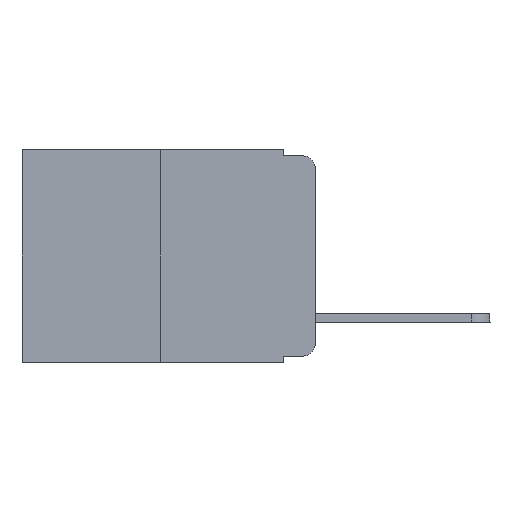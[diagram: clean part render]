
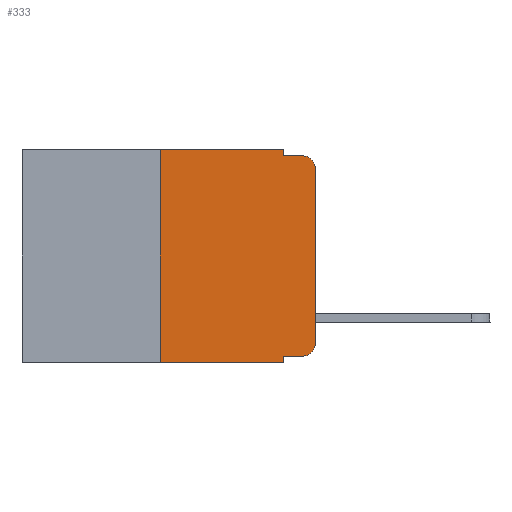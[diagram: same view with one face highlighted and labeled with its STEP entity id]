
A CAD part, left-side view. The second image highlights one B-rep face of the part: STEP entity #333.
In plain terms, the highlighted planar face has unit normal (-1, 0, 0).
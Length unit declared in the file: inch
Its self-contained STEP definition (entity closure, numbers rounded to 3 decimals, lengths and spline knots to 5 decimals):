
#112 = LINE ( 'NONE', #10300, #6305 ) ;
#148 = CARTESIAN_POINT ( 'NONE',  ( 0., 0.473, 0. ) ) ;
#184 = CARTESIAN_POINT ( 'NONE',  ( 0., 0.02, -0.313 ) ) ;
#333 = ADVANCED_FACE ( 'NONE', ( #2467 ), #12265, .F. ) ;
#410 = VECTOR ( 'NONE', #12248, 39.37008 ) ;
#501 = EDGE_CURVE ( 'NONE', #10799, #5024, #112, .T. ) ;
#825 = VECTOR ( 'NONE', #7896, 39.37008 ) ;
#920 = EDGE_CURVE ( 'NONE', #13143, #12940, #6471, .T. ) ;
#958 = CARTESIAN_POINT ( 'NONE',  ( 0., 0.02, -0.333 ) ) ;
#990 = DIRECTION ( 'NONE',  ( 0., 0., -1. ) ) ;
#1662 = LINE ( 'NONE', #13564, #9919 ) ;
#1767 = VERTEX_POINT ( 'NONE', #10139 ) ;
#1808 = CIRCLE ( 'NONE', #14668, 0.02 ) ;
#1961 = CARTESIAN_POINT ( 'NONE',  ( 0., 0.051, -0.01 ) ) ;
#2074 = ORIENTED_EDGE ( 'NONE', *, *, #2558, .T. ) ;
#2287 = VERTEX_POINT ( 'NONE', #15857 ) ;
#2348 = EDGE_CURVE ( 'NONE', #12079, #1767, #2848, .T. ) ;
#2377 = CIRCLE ( 'NONE', #14820, 0.02 ) ;
#2427 = LINE ( 'NONE', #7801, #11066 ) ;
#2467 = FACE_OUTER_BOUND ( 'NONE', #6230, .T. ) ;
#2558 = EDGE_CURVE ( 'NONE', #12079, #7260, #1662, .T. ) ;
#2848 = LINE ( 'NONE', #14008, #4174 ) ;
#3123 = DIRECTION ( 'NONE',  ( 0., 0., -1. ) ) ;
#3157 = LINE ( 'NONE', #14130, #825 ) ;
#3740 = LINE ( 'NONE', #7368, #410 ) ;
#3996 = DIRECTION ( 'NONE',  ( 0., 0., -1. ) ) ;
#4174 = VECTOR ( 'NONE', #10405, 39.37008 ) ;
#4663 = EDGE_CURVE ( 'NONE', #2287, #5148, #3157, .T. ) ;
#4719 = CARTESIAN_POINT ( 'NONE',  ( 0., 0.02, -0.03 ) ) ;
#4754 = VECTOR ( 'NONE', #7953, 39.37008 ) ;
#4758 = EDGE_CURVE ( 'NONE', #12940, #11638, #2377, .T. ) ;
#4834 = CARTESIAN_POINT ( 'NONE',  ( 0., 0., -0.03 ) ) ;
#4956 = AXIS2_PLACEMENT_3D ( 'NONE', #148, #6360, #8750 ) ;
#5024 = VERTEX_POINT ( 'NONE', #1961 ) ;
#5148 = VERTEX_POINT ( 'NONE', #958 ) ;
#5492 = CARTESIAN_POINT ( 'NONE',  ( 0., 0., -0.313 ) ) ;
#6230 = EDGE_LOOP ( 'NONE', ( #7452, #14135, #14355, #7091, #9943, #14234, #2074, #13016, #6827, #6243 ) ) ;
#6243 = ORIENTED_EDGE ( 'NONE', *, *, #8329, .T. ) ;
#6305 = VECTOR ( 'NONE', #3123, 39.37008 ) ;
#6360 = DIRECTION ( 'NONE',  ( 1., 0., 0. ) ) ;
#6457 = DIRECTION ( 'NONE',  ( -1., 0., 0. ) ) ;
#6471 = LINE ( 'NONE', #14773, #12975 ) ;
#6547 = CARTESIAN_POINT ( 'NONE',  ( 0., 0.051, 0. ) ) ;
#6637 = DIRECTION ( 'NONE',  ( 0., -1., 0. ) ) ;
#6827 = ORIENTED_EDGE ( 'NONE', *, *, #4663, .T. ) ;
#7091 = ORIENTED_EDGE ( 'NONE', *, *, #501, .F. ) ;
#7243 = LINE ( 'NONE', #6547, #4754 ) ;
#7260 = VERTEX_POINT ( 'NONE', #10378 ) ;
#7368 = CARTESIAN_POINT ( 'NONE',  ( 0., 0.051, -0.01 ) ) ;
#7452 = ORIENTED_EDGE ( 'NONE', *, *, #920, .T. ) ;
#7801 = CARTESIAN_POINT ( 'NONE',  ( 0., 0.473, 0. ) ) ;
#7896 = DIRECTION ( 'NONE',  ( 0., -1., 0. ) ) ;
#7953 = DIRECTION ( 'NONE',  ( 0., 0., -1. ) ) ;
#8093 = CARTESIAN_POINT ( 'NONE',  ( 0., 0.02, -0.01 ) ) ;
#8329 = EDGE_CURVE ( 'NONE', #5148, #13143, #1808, .T. ) ;
#8678 = EDGE_CURVE ( 'NONE', #5024, #11638, #3740, .T. ) ;
#8750 = DIRECTION ( 'NONE',  ( 0., 0., -1. ) ) ;
#9919 = VECTOR ( 'NONE', #10283, 39.37008 ) ;
#9943 = ORIENTED_EDGE ( 'NONE', *, *, #12693, .F. ) ;
#10139 = CARTESIAN_POINT ( 'NONE',  ( 0., 0.25, 0. ) ) ;
#10283 = DIRECTION ( 'NONE',  ( 0., -1., 0. ) ) ;
#10300 = CARTESIAN_POINT ( 'NONE',  ( 0., 0.051, 0. ) ) ;
#10378 = CARTESIAN_POINT ( 'NONE',  ( 0., 0.051, -0.343 ) ) ;
#10405 = DIRECTION ( 'NONE',  ( 0., 0., 1. ) ) ;
#10799 = VERTEX_POINT ( 'NONE', #13508 ) ;
#11066 = VECTOR ( 'NONE', #6637, 39.37008 ) ;
#11638 = VERTEX_POINT ( 'NONE', #8093 ) ;
#12079 = VERTEX_POINT ( 'NONE', #15041 ) ;
#12248 = DIRECTION ( 'NONE',  ( 0., -1., 0. ) ) ;
#12265 = PLANE ( 'NONE',  #4956 ) ;
#12580 = EDGE_CURVE ( 'NONE', #2287, #7260, #7243, .T. ) ;
#12693 = EDGE_CURVE ( 'NONE', #1767, #10799, #2427, .T. ) ;
#12940 = VERTEX_POINT ( 'NONE', #4834 ) ;
#12975 = VECTOR ( 'NONE', #15877, 39.37008 ) ;
#13016 = ORIENTED_EDGE ( 'NONE', *, *, #12580, .F. ) ;
#13143 = VERTEX_POINT ( 'NONE', #5492 ) ;
#13508 = CARTESIAN_POINT ( 'NONE',  ( 0., 0.051, 0. ) ) ;
#13564 = CARTESIAN_POINT ( 'NONE',  ( 0., 0.473, -0.343 ) ) ;
#14008 = CARTESIAN_POINT ( 'NONE',  ( 0., 0.25, 0. ) ) ;
#14130 = CARTESIAN_POINT ( 'NONE',  ( 0., 0.051, -0.333 ) ) ;
#14135 = ORIENTED_EDGE ( 'NONE', *, *, #4758, .T. ) ;
#14234 = ORIENTED_EDGE ( 'NONE', *, *, #2348, .F. ) ;
#14355 = ORIENTED_EDGE ( 'NONE', *, *, #8678, .F. ) ;
#14668 = AXIS2_PLACEMENT_3D ( 'NONE', #184, #6457, #3996 ) ;
#14773 = CARTESIAN_POINT ( 'NONE',  ( 0., 0., 0. ) ) ;
#14820 = AXIS2_PLACEMENT_3D ( 'NONE', #4719, #15750, #990 ) ;
#15041 = CARTESIAN_POINT ( 'NONE',  ( 0., 0.25, -0.343 ) ) ;
#15750 = DIRECTION ( 'NONE',  ( -1., 0., 0. ) ) ;
#15857 = CARTESIAN_POINT ( 'NONE',  ( 0., 0.051, -0.333 ) ) ;
#15877 = DIRECTION ( 'NONE',  ( 0., 0., 1. ) ) ;
